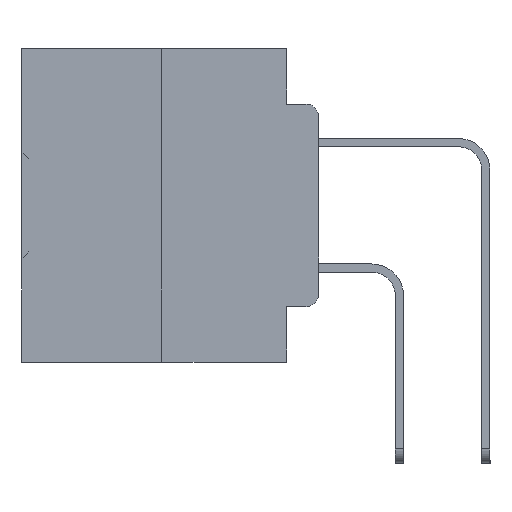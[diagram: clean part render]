
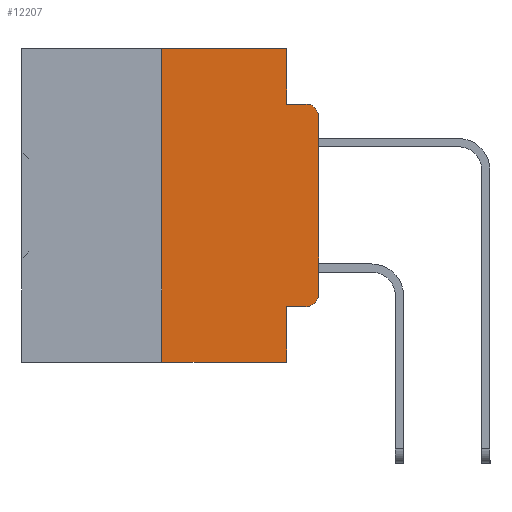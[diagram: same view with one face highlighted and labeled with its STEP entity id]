
A CAD part, left-side view. The second image highlights one B-rep face of the part: STEP entity #12207.
In plain terms, the highlighted planar face has unit normal (-1, 0, 0).
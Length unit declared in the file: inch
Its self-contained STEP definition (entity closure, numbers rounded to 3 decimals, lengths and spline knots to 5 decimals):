
#220 = CARTESIAN_POINT ( 'NONE',  ( 0., 0.02, -0.1085 ) ) ;
#290 = CARTESIAN_POINT ( 'NONE',  ( 0., 0.051, 0. ) ) ;
#1295 = VECTOR ( 'NONE', #34711, 39.37008 ) ;
#1404 = CARTESIAN_POINT ( 'NONE',  ( 0., 0.02, -0.4115 ) ) ;
#1590 = ORIENTED_EDGE ( 'NONE', *, *, #30974, .F. ) ;
#1680 = CARTESIAN_POINT ( 'NONE',  ( 0., 0., -0.3915 ) ) ;
#3109 = ORIENTED_EDGE ( 'NONE', *, *, #13427, .T. ) ;
#3406 = DIRECTION ( 'NONE',  ( 0., 0., -1. ) ) ;
#4560 = LINE ( 'NONE', #19570, #19310 ) ;
#5035 = EDGE_CURVE ( 'NONE', #35552, #28917, #27644, .T. ) ;
#5499 = AXIS2_PLACEMENT_3D ( 'NONE', #26549, #7802, #29659 ) ;
#6950 = ORIENTED_EDGE ( 'NONE', *, *, #37141, .F. ) ;
#7136 = EDGE_CURVE ( 'NONE', #28979, #28917, #12306, .T. ) ;
#7802 = DIRECTION ( 'NONE',  ( 1., 0., 0. ) ) ;
#8044 = LINE ( 'NONE', #14709, #31022 ) ;
#8193 = EDGE_LOOP ( 'NONE', ( #3109, #13058, #12740, #6950, #9132, #24034, #9793, #1590, #10316, #21311 ) ) ;
#8425 = VERTEX_POINT ( 'NONE', #16473 ) ;
#8951 = CARTESIAN_POINT ( 'NONE',  ( 0., 0.051, -0.4115 ) ) ;
#8987 = CARTESIAN_POINT ( 'NONE',  ( 0., 0.051, -0.5 ) ) ;
#9132 = ORIENTED_EDGE ( 'NONE', *, *, #36677, .F. ) ;
#9340 = VERTEX_POINT ( 'NONE', #8987 ) ;
#9712 = CARTESIAN_POINT ( 'NONE',  ( 0., 0.25, 0. ) ) ;
#9731 = VERTEX_POINT ( 'NONE', #1404 ) ;
#9748 = DIRECTION ( 'NONE',  ( 0., 0., -1. ) ) ;
#9793 = ORIENTED_EDGE ( 'NONE', *, *, #18226, .T. ) ;
#10316 = ORIENTED_EDGE ( 'NONE', *, *, #26822, .T. ) ;
#10567 = CIRCLE ( 'NONE', #28712, 0.02 ) ;
#11008 = DIRECTION ( 'NONE',  ( -1., 0., 0. ) ) ;
#11102 = VECTOR ( 'NONE', #22228, 39.37008 ) ;
#12207 = ADVANCED_FACE ( 'NONE', ( #12582 ), #13959, .F. ) ;
#12306 = CIRCLE ( 'NONE', #24524, 0.02 ) ;
#12582 = FACE_OUTER_BOUND ( 'NONE', #8193, .T. ) ;
#12740 = ORIENTED_EDGE ( 'NONE', *, *, #5035, .F. ) ;
#13058 = ORIENTED_EDGE ( 'NONE', *, *, #7136, .T. ) ;
#13379 = VECTOR ( 'NONE', #9748, 39.37008 ) ;
#13427 = EDGE_CURVE ( 'NONE', #22078, #28979, #19370, .T. ) ;
#13765 = CARTESIAN_POINT ( 'NONE',  ( 0., 0., 0. ) ) ;
#13959 = PLANE ( 'NONE',  #5499 ) ;
#14709 = CARTESIAN_POINT ( 'NONE',  ( 0., 0.473, 0. ) ) ;
#15951 = CARTESIAN_POINT ( 'NONE',  ( 0., 0.051, 0. ) ) ;
#16473 = CARTESIAN_POINT ( 'NONE',  ( 0., 0.051, 0. ) ) ;
#18226 = EDGE_CURVE ( 'NONE', #19418, #9340, #4560, .T. ) ;
#18591 = CARTESIAN_POINT ( 'NONE',  ( 0., 0., -0.1085 ) ) ;
#19310 = VECTOR ( 'NONE', #22693, 39.37008 ) ;
#19370 = LINE ( 'NONE', #13765, #35867 ) ;
#19418 = VERTEX_POINT ( 'NONE', #38237 ) ;
#19455 = LINE ( 'NONE', #15951, #11102 ) ;
#19570 = CARTESIAN_POINT ( 'NONE',  ( 0., 0.473, -0.5 ) ) ;
#20115 = DIRECTION ( 'NONE',  ( 0., 0., 1. ) ) ;
#20787 = VECTOR ( 'NONE', #30833, 39.37008 ) ;
#21311 = ORIENTED_EDGE ( 'NONE', *, *, #24727, .T. ) ;
#21685 = CARTESIAN_POINT ( 'NONE',  ( 0., 0.25, 0. ) ) ;
#22078 = VERTEX_POINT ( 'NONE', #1680 ) ;
#22184 = DIRECTION ( 'NONE',  ( -1., 0., 0. ) ) ;
#22228 = DIRECTION ( 'NONE',  ( 0., 0., -1. ) ) ;
#22693 = DIRECTION ( 'NONE',  ( 0., -1., 0. ) ) ;
#23085 = VERTEX_POINT ( 'NONE', #21685 ) ;
#24034 = ORIENTED_EDGE ( 'NONE', *, *, #35111, .F. ) ;
#24524 = AXIS2_PLACEMENT_3D ( 'NONE', #220, #22184, #3406 ) ;
#24712 = CARTESIAN_POINT ( 'NONE',  ( 0., 0.051, -0.4115 ) ) ;
#24727 = EDGE_CURVE ( 'NONE', #9731, #22078, #10567, .T. ) ;
#26306 = LINE ( 'NONE', #9712, #1295 ) ;
#26549 = CARTESIAN_POINT ( 'NONE',  ( 0., 0.473, 0. ) ) ;
#26822 = EDGE_CURVE ( 'NONE', #26830, #9731, #30029, .T. ) ;
#26830 = VERTEX_POINT ( 'NONE', #24712 ) ;
#27644 = LINE ( 'NONE', #33775, #34923 ) ;
#28712 = AXIS2_PLACEMENT_3D ( 'NONE', #29715, #11008, #32859 ) ;
#28917 = VERTEX_POINT ( 'NONE', #33823 ) ;
#28979 = VERTEX_POINT ( 'NONE', #18591 ) ;
#29659 = DIRECTION ( 'NONE',  ( 0., 0., -1. ) ) ;
#29715 = CARTESIAN_POINT ( 'NONE',  ( 0., 0.02, -0.3915 ) ) ;
#30022 = LINE ( 'NONE', #290, #13379 ) ;
#30029 = LINE ( 'NONE', #8951, #20787 ) ;
#30653 = DIRECTION ( 'NONE',  ( 0., -1., 0. ) ) ;
#30833 = DIRECTION ( 'NONE',  ( 0., -1., 0. ) ) ;
#30974 = EDGE_CURVE ( 'NONE', #26830, #9340, #19455, .T. ) ;
#31022 = VECTOR ( 'NONE', #36449, 39.37008 ) ;
#32859 = DIRECTION ( 'NONE',  ( 0., 0., -1. ) ) ;
#33775 = CARTESIAN_POINT ( 'NONE',  ( 0., 0.051, -0.0885 ) ) ;
#33823 = CARTESIAN_POINT ( 'NONE',  ( 0., 0.02, -0.0885 ) ) ;
#34146 = CARTESIAN_POINT ( 'NONE',  ( 0., 0.051, -0.0885 ) ) ;
#34711 = DIRECTION ( 'NONE',  ( 0., 0., 1. ) ) ;
#34923 = VECTOR ( 'NONE', #30653, 39.37008 ) ;
#35111 = EDGE_CURVE ( 'NONE', #19418, #23085, #26306, .T. ) ;
#35552 = VERTEX_POINT ( 'NONE', #34146 ) ;
#35867 = VECTOR ( 'NONE', #20115, 39.37008 ) ;
#36449 = DIRECTION ( 'NONE',  ( 0., -1., 0. ) ) ;
#36677 = EDGE_CURVE ( 'NONE', #23085, #8425, #8044, .T. ) ;
#37141 = EDGE_CURVE ( 'NONE', #8425, #35552, #30022, .T. ) ;
#38237 = CARTESIAN_POINT ( 'NONE',  ( 0., 0.25, -0.5 ) ) ;
